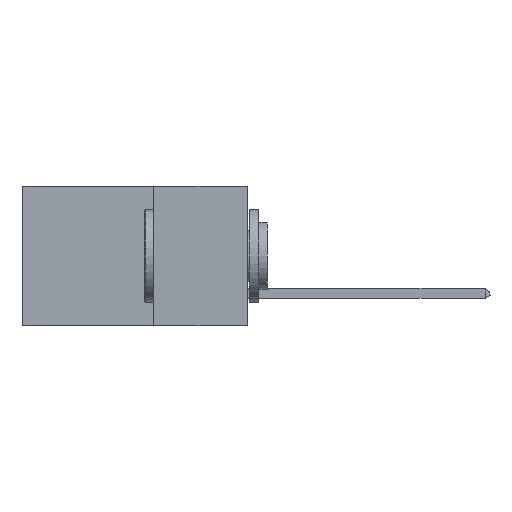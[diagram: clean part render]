
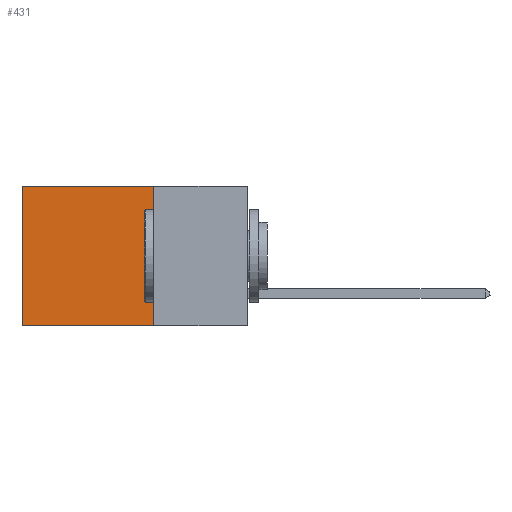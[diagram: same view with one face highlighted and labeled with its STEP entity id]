
A CAD part, left-side view. The second image highlights one B-rep face of the part: STEP entity #431.
In plain terms, the highlighted planar face has unit normal (-1, 0, 0).
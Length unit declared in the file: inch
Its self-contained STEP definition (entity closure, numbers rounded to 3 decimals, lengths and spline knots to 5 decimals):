
#431 = ADVANCED_FACE ( 'NONE', ( #26615 ), #28040, .F. ) ;
#1849 = DIRECTION ( 'NONE',  ( 0., 1., 0. ) ) ;
#3327 = ORIENTED_EDGE ( 'NONE', *, *, #4708, .F. ) ;
#4708 = EDGE_CURVE ( 'NONE', #11850, #25781, #28955, .T. ) ;
#4739 = VERTEX_POINT ( 'NONE', #13874 ) ;
#4989 = EDGE_LOOP ( 'NONE', ( #24163, #16170, #3327, #10278 ) ) ;
#5200 = DIRECTION ( 'NONE',  ( 0., 0., -1. ) ) ;
#5475 = CARTESIAN_POINT ( 'NONE',  ( 0.298, 0.25, -0.37 ) ) ;
#6085 = AXIS2_PLACEMENT_3D ( 'NONE', #6921, #14240, #14036 ) ;
#6921 = CARTESIAN_POINT ( 'NONE',  ( 0.298, 0.25, 0. ) ) ;
#7448 = LINE ( 'NONE', #27516, #29662 ) ;
#7918 = CARTESIAN_POINT ( 'NONE',  ( 0.298, 0.25, 0. ) ) ;
#10278 = ORIENTED_EDGE ( 'NONE', *, *, #29972, .T. ) ;
#10752 = CARTESIAN_POINT ( 'NONE',  ( 0.298, 0.6, 0. ) ) ;
#11850 = VERTEX_POINT ( 'NONE', #7918 ) ;
#13569 = VERTEX_POINT ( 'NONE', #10752 ) ;
#13874 = CARTESIAN_POINT ( 'NONE',  ( 0.298, 0.6, -0.37 ) ) ;
#14036 = DIRECTION ( 'NONE',  ( 0., 0., -1. ) ) ;
#14240 = DIRECTION ( 'NONE',  ( 1., 0., 0. ) ) ;
#14714 = VECTOR ( 'NONE', #1849, 39.37008 ) ;
#16170 = ORIENTED_EDGE ( 'NONE', *, *, #27833, .F. ) ;
#18266 = DIRECTION ( 'NONE',  ( 0., 1., 0. ) ) ;
#19320 = CARTESIAN_POINT ( 'NONE',  ( 0.298, 0.6, 0. ) ) ;
#19873 = EDGE_CURVE ( 'NONE', #13569, #4739, #25365, .T. ) ;
#23038 = VECTOR ( 'NONE', #27972, 39.37008 ) ;
#24163 = ORIENTED_EDGE ( 'NONE', *, *, #19873, .T. ) ;
#25365 = LINE ( 'NONE', #19320, #29760 ) ;
#25613 = CARTESIAN_POINT ( 'NONE',  ( 0.298, 0.25, 0. ) ) ;
#25781 = VERTEX_POINT ( 'NONE', #5475 ) ;
#26615 = FACE_OUTER_BOUND ( 'NONE', #4989, .T. ) ;
#27516 = CARTESIAN_POINT ( 'NONE',  ( 0.298, 0.25, -0.37 ) ) ;
#27812 = CARTESIAN_POINT ( 'NONE',  ( 0.298, 0.25, 0. ) ) ;
#27833 = EDGE_CURVE ( 'NONE', #25781, #4739, #7448, .T. ) ;
#27972 = DIRECTION ( 'NONE',  ( 0., 0., -1. ) ) ;
#28040 = PLANE ( 'NONE',  #6085 ) ;
#28443 = LINE ( 'NONE', #27812, #14714 ) ;
#28955 = LINE ( 'NONE', #25613, #23038 ) ;
#29662 = VECTOR ( 'NONE', #18266, 39.37008 ) ;
#29760 = VECTOR ( 'NONE', #5200, 39.37008 ) ;
#29972 = EDGE_CURVE ( 'NONE', #11850, #13569, #28443, .T. ) ;
